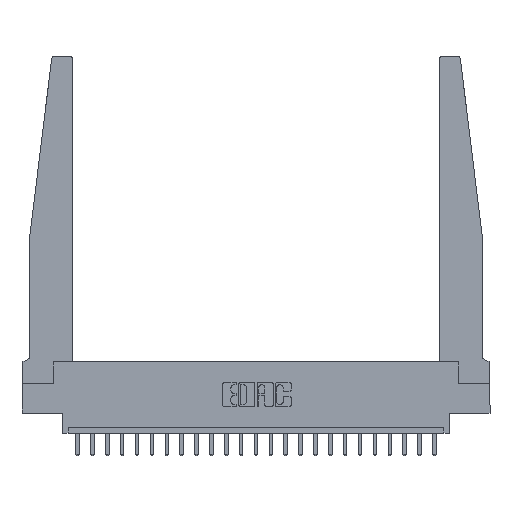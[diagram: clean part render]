
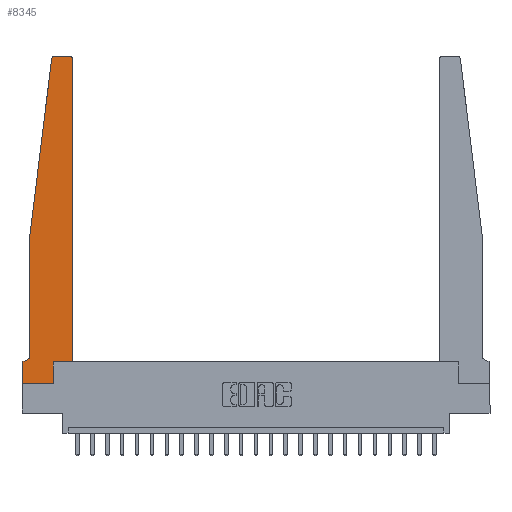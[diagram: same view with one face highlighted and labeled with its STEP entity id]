
A CAD part, top view. The second image highlights one B-rep face of the part: STEP entity #8345.
In plain terms, the highlighted planar face has unit normal (0, 0, 1).
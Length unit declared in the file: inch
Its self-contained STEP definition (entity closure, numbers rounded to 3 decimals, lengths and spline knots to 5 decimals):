
#140 = VECTOR ( 'NONE', #2682, 39.37008 ) ;
#628 = CARTESIAN_POINT ( 'NONE',  ( 0.065, 1.25, 0.37 ) ) ;
#631 = AXIS2_PLACEMENT_3D ( 'NONE', #15824, #14139, #12364 ) ;
#666 = DIRECTION ( 'NONE',  ( -1., 0., 0. ) ) ;
#1268 = EDGE_CURVE ( 'NONE', #21591, #6115, #13404, .T. ) ;
#1619 = CARTESIAN_POINT ( 'NONE',  ( 0.065, 0.1875, 0.37 ) ) ;
#2063 = EDGE_CURVE ( 'NONE', #6115, #6386, #15836, .T. ) ;
#2566 = VECTOR ( 'NONE', #14076, 39.37008 ) ;
#2682 = DIRECTION ( 'NONE',  ( 1., 0., 0. ) ) ;
#2737 = ORIENTED_EDGE ( 'NONE', *, *, #14175, .T. ) ;
#2747 = VERTEX_POINT ( 'NONE', #5353 ) ;
#2961 = ORIENTED_EDGE ( 'NONE', *, *, #7195, .T. ) ;
#3018 = DIRECTION ( 'NONE',  ( 1., 0., 0. ) ) ;
#3108 = VERTEX_POINT ( 'NONE', #21380 ) ;
#3144 = AXIS2_PLACEMENT_3D ( 'NONE', #21396, #5775, #14289 ) ;
#3252 = VERTEX_POINT ( 'NONE', #12793 ) ;
#3306 = EDGE_CURVE ( 'NONE', #3346, #21591, #21897, .T. ) ;
#3346 = VERTEX_POINT ( 'NONE', #3348 ) ;
#3348 = CARTESIAN_POINT ( 'NONE',  ( 0.425, 2.72, 0.37 ) ) ;
#3719 = LINE ( 'NONE', #13031, #140 ) ;
#3756 = LINE ( 'NONE', #13745, #4311 ) ;
#3849 = LINE ( 'NONE', #15216, #6056 ) ;
#3879 = VECTOR ( 'NONE', #18203, 39.37008 ) ;
#4311 = VECTOR ( 'NONE', #18634, 39.37008 ) ;
#4692 = LINE ( 'NONE', #11104, #3879 ) ;
#4898 = VERTEX_POINT ( 'NONE', #19299 ) ;
#5353 = CARTESIAN_POINT ( 'NONE',  ( 0.2605, 0., 0.37 ) ) ;
#5538 = ORIENTED_EDGE ( 'NONE', *, *, #9882, .T. ) ;
#5740 = ORIENTED_EDGE ( 'NONE', *, *, #1268, .T. ) ;
#5775 = DIRECTION ( 'NONE',  ( 0., 0., 1. ) ) ;
#5801 = CARTESIAN_POINT ( 'NONE',  ( 0.2605, 0.18, 0.37 ) ) ;
#6056 = VECTOR ( 'NONE', #16977, 39.37008 ) ;
#6063 = CARTESIAN_POINT ( 'NONE',  ( 0.24675, 2.72367, 0.37 ) ) ;
#6115 = VERTEX_POINT ( 'NONE', #12492 ) ;
#6386 = VERTEX_POINT ( 'NONE', #6063 ) ;
#6632 = CIRCLE ( 'NONE', #13852, 0.05 ) ;
#6948 = EDGE_CURVE ( 'NONE', #22350, #3252, #4692, .T. ) ;
#7047 = ORIENTED_EDGE ( 'NONE', *, *, #3306, .T. ) ;
#7195 = EDGE_CURVE ( 'NONE', #3252, #9292, #6632, .T. ) ;
#7793 = CARTESIAN_POINT ( 'NONE',  ( 0.065, 1.25, 0.37 ) ) ;
#7927 = VECTOR ( 'NONE', #12970, 39.37008 ) ;
#8194 = AXIS2_PLACEMENT_3D ( 'NONE', #11724, #15333, #3018 ) ;
#8345 = ADVANCED_FACE ( 'NONE', ( #22583 ), #16784, .T. ) ;
#8369 = ORIENTED_EDGE ( 'NONE', *, *, #2063, .T. ) ;
#8811 = EDGE_CURVE ( 'NONE', #4898, #3346, #18402, .T. ) ;
#8983 = DIRECTION ( 'NONE',  ( -1., 0., 0. ) ) ;
#9292 = VERTEX_POINT ( 'NONE', #13049 ) ;
#9497 = EDGE_CURVE ( 'NONE', #17059, #3108, #3756, .T. ) ;
#9882 = EDGE_CURVE ( 'NONE', #9292, #17059, #10619, .T. ) ;
#10544 = ORIENTED_EDGE ( 'NONE', *, *, #6948, .T. ) ;
#10619 = LINE ( 'NONE', #1619, #19478 ) ;
#10851 = CARTESIAN_POINT ( 'NONE',  ( 0., 0.1875, 0.37 ) ) ;
#11065 = EDGE_CURVE ( 'NONE', #6386, #22350, #12040, .T. ) ;
#11104 = CARTESIAN_POINT ( 'NONE',  ( 0.065, 1.25, 0.37 ) ) ;
#11724 = CARTESIAN_POINT ( 'NONE',  ( 0., 0.1875, 0.37 ) ) ;
#12040 = LINE ( 'NONE', #628, #7927 ) ;
#12326 = CARTESIAN_POINT ( 'NONE',  ( 0.015, 0.2375, 0.37 ) ) ;
#12364 = DIRECTION ( 'NONE',  ( 1., 0., 0. ) ) ;
#12492 = CARTESIAN_POINT ( 'NONE',  ( 0.27653, 2.75, 0.37 ) ) ;
#12753 = EDGE_CURVE ( 'NONE', #21220, #4898, #3719, .T. ) ;
#12793 = CARTESIAN_POINT ( 'NONE',  ( 0.065, 0.2375, 0.37 ) ) ;
#12970 = DIRECTION ( 'NONE',  ( -0.122, -0.992, 0. ) ) ;
#13031 = CARTESIAN_POINT ( 'NONE',  ( 0.425, 0.18, 0.37 ) ) ;
#13049 = CARTESIAN_POINT ( 'NONE',  ( 0.015, 0.1875, 0.37 ) ) ;
#13301 = DIRECTION ( 'NONE',  ( 0., 1., 0. ) ) ;
#13404 = LINE ( 'NONE', #20124, #18638 ) ;
#13725 = VECTOR ( 'NONE', #13301, 39.37008 ) ;
#13745 = CARTESIAN_POINT ( 'NONE',  ( 0., 0., 0.37 ) ) ;
#13852 = AXIS2_PLACEMENT_3D ( 'NONE', #12326, #17634, #19133 ) ;
#14076 = DIRECTION ( 'NONE',  ( 1., 0., 0. ) ) ;
#14139 = DIRECTION ( 'NONE',  ( 0., 0., 1. ) ) ;
#14175 = EDGE_CURVE ( 'NONE', #3108, #2747, #18294, .T. ) ;
#14289 = DIRECTION ( 'NONE',  ( 1., 0., 0. ) ) ;
#14773 = ORIENTED_EDGE ( 'NONE', *, *, #15971, .T. ) ;
#14777 = ORIENTED_EDGE ( 'NONE', *, *, #11065, .T. ) ;
#15216 = CARTESIAN_POINT ( 'NONE',  ( 0.2605, 0.18, 0.37 ) ) ;
#15333 = DIRECTION ( 'NONE',  ( 0., 0., 1. ) ) ;
#15824 = CARTESIAN_POINT ( 'NONE',  ( 0.395, 2.72, 0.37 ) ) ;
#15836 = CIRCLE ( 'NONE', #3144, 0.03 ) ;
#15971 = EDGE_CURVE ( 'NONE', #2747, #21220, #3849, .T. ) ;
#16784 = PLANE ( 'NONE',  #8194 ) ;
#16977 = DIRECTION ( 'NONE',  ( 0., 1., 0. ) ) ;
#17059 = VERTEX_POINT ( 'NONE', #10851 ) ;
#17431 = CARTESIAN_POINT ( 'NONE',  ( 0., 0., 0.37 ) ) ;
#17634 = DIRECTION ( 'NONE',  ( 0., 0., -1. ) ) ;
#18203 = DIRECTION ( 'NONE',  ( 0., -1., 0. ) ) ;
#18294 = LINE ( 'NONE', #17431, #2566 ) ;
#18402 = LINE ( 'NONE', #22399, #13725 ) ;
#18634 = DIRECTION ( 'NONE',  ( 0., -1., 0. ) ) ;
#18638 = VECTOR ( 'NONE', #666, 39.37008 ) ;
#19133 = DIRECTION ( 'NONE',  ( -1., 0., 0. ) ) ;
#19299 = CARTESIAN_POINT ( 'NONE',  ( 0.425, 0.18, 0.37 ) ) ;
#19478 = VECTOR ( 'NONE', #8983, 39.37008 ) ;
#20124 = CARTESIAN_POINT ( 'NONE',  ( 0.25, 2.75, 0.37 ) ) ;
#20351 = ORIENTED_EDGE ( 'NONE', *, *, #8811, .T. ) ;
#20684 = EDGE_LOOP ( 'NONE', ( #5740, #8369, #14777, #10544, #2961, #5538, #20872, #2737, #14773, #22774, #20351, #7047 ) ) ;
#20858 = CARTESIAN_POINT ( 'NONE',  ( 0.395, 2.75, 0.37 ) ) ;
#20872 = ORIENTED_EDGE ( 'NONE', *, *, #9497, .T. ) ;
#21220 = VERTEX_POINT ( 'NONE', #5801 ) ;
#21380 = CARTESIAN_POINT ( 'NONE',  ( 0., 0., 0.37 ) ) ;
#21396 = CARTESIAN_POINT ( 'NONE',  ( 0.27653, 2.72, 0.37 ) ) ;
#21591 = VERTEX_POINT ( 'NONE', #20858 ) ;
#21897 = CIRCLE ( 'NONE', #631, 0.03 ) ;
#22350 = VERTEX_POINT ( 'NONE', #7793 ) ;
#22399 = CARTESIAN_POINT ( 'NONE',  ( 0.425, 0.18, 0.37 ) ) ;
#22583 = FACE_OUTER_BOUND ( 'NONE', #20684, .T. ) ;
#22774 = ORIENTED_EDGE ( 'NONE', *, *, #12753, .T. ) ;
